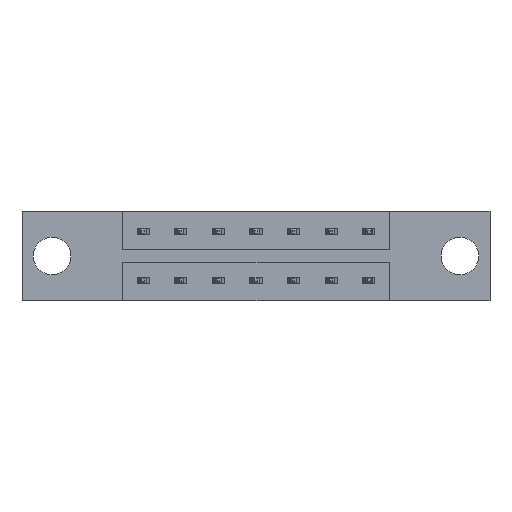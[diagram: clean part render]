
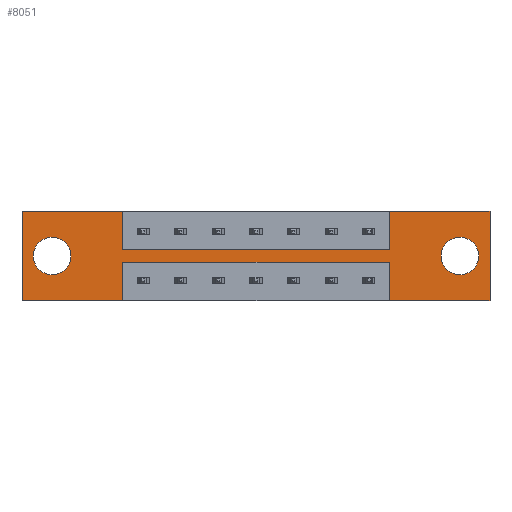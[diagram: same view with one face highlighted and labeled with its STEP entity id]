
A CAD part, front view. The second image highlights one B-rep face of the part: STEP entity #8051.
In plain terms, the highlighted planar face has unit normal (0, -1, 0).
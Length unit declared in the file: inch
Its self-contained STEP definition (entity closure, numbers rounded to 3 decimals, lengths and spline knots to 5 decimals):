
#23 = DIRECTION ( 'NONE',  ( 0., 0., 1. ) ) ;
#122 = DIRECTION ( 'NONE',  ( -1., 0., 0. ) ) ;
#173 = ORIENTED_EDGE ( 'NONE', *, *, #7002, .T. ) ;
#308 = VERTEX_POINT ( 'NONE', #1861 ) ;
#310 = ORIENTED_EDGE ( 'NONE', *, *, #7567, .F. ) ;
#315 = DIRECTION ( 'NONE',  ( 0., 1., 0. ) ) ;
#384 = EDGE_CURVE ( 'NONE', #308, #1176, #7530, .T. ) ;
#392 = ORIENTED_EDGE ( 'NONE', *, *, #9066, .T. ) ;
#439 = VERTEX_POINT ( 'NONE', #3459 ) ;
#445 = EDGE_CURVE ( 'NONE', #5451, #8103, #5532, .T. ) ;
#446 = ORIENTED_EDGE ( 'NONE', *, *, #5977, .F. ) ;
#511 = CIRCLE ( 'NONE', #1690, 0.078 ) ;
#558 = VECTOR ( 'NONE', #1764, 39.37008 ) ;
#586 = LINE ( 'NONE', #7696, #5317 ) ;
#608 = CARTESIAN_POINT ( 'NONE',  ( 0.4175, 0., -0.1585 ) ) ;
#742 = CARTESIAN_POINT ( 'NONE',  ( 0., 0., -0.37 ) ) ;
#937 = CIRCLE ( 'NONE', #1239, 0.078 ) ;
#938 = EDGE_CURVE ( 'NONE', #2151, #2576, #6186, .T. ) ;
#1021 = DIRECTION ( 'NONE',  ( 0., 0., -1. ) ) ;
#1129 = VECTOR ( 'NONE', #5415, 39.37008 ) ;
#1176 = VERTEX_POINT ( 'NONE', #1237 ) ;
#1177 = ORIENTED_EDGE ( 'NONE', *, *, #445, .T. ) ;
#1206 = CARTESIAN_POINT ( 'NONE',  ( 0., 0., -0.37 ) ) ;
#1237 = CARTESIAN_POINT ( 'NONE',  ( 0.4175, 0., -0.1585 ) ) ;
#1239 = AXIS2_PLACEMENT_3D ( 'NONE', #5053, #7260, #5105 ) ;
#1272 = EDGE_CURVE ( 'NONE', #8853, #7526, #586, .T. ) ;
#1282 = ORIENTED_EDGE ( 'NONE', *, *, #1272, .F. ) ;
#1418 = CARTESIAN_POINT ( 'NONE',  ( 1.815, 0., -0.263 ) ) ;
#1430 = EDGE_LOOP ( 'NONE', ( #7044, #6450, #446, #1282, #3227, #310, #8254, #4427, #1470, #2848, #5745, #5926 ) ) ;
#1470 = ORIENTED_EDGE ( 'NONE', *, *, #1856, .F. ) ;
#1485 = CARTESIAN_POINT ( 'NONE',  ( 0.4175, 0., -0.2115 ) ) ;
#1657 = LINE ( 'NONE', #1485, #8416 ) ;
#1690 = AXIS2_PLACEMENT_3D ( 'NONE', #4483, #315, #1021 ) ;
#1727 = VECTOR ( 'NONE', #122, 39.37008 ) ;
#1764 = DIRECTION ( 'NONE',  ( 0., 0., 1. ) ) ;
#1856 = EDGE_CURVE ( 'NONE', #7547, #3653, #6992, .T. ) ;
#1861 = CARTESIAN_POINT ( 'NONE',  ( 0.4175, 0., 0. ) ) ;
#2132 = LINE ( 'NONE', #5685, #6355 ) ;
#2151 = VERTEX_POINT ( 'NONE', #3262 ) ;
#2155 = CARTESIAN_POINT ( 'NONE',  ( 0., 0., -0.37 ) ) ;
#2385 = LINE ( 'NONE', #5078, #8700 ) ;
#2402 = CARTESIAN_POINT ( 'NONE',  ( 0.4175, 0., -0.2115 ) ) ;
#2416 = CARTESIAN_POINT ( 'NONE',  ( 1.815, 0., -0.107 ) ) ;
#2446 = LINE ( 'NONE', #2402, #8591 ) ;
#2576 = VERTEX_POINT ( 'NONE', #5306 ) ;
#2579 = LINE ( 'NONE', #8041, #558 ) ;
#2848 = ORIENTED_EDGE ( 'NONE', *, *, #4275, .F. ) ;
#2861 = CARTESIAN_POINT ( 'NONE',  ( 1.5225, 0., 0. ) ) ;
#2882 = PLANE ( 'NONE',  #6802 ) ;
#2903 = EDGE_CURVE ( 'NONE', #3653, #308, #2385, .T. ) ;
#2936 = LINE ( 'NONE', #6287, #6354 ) ;
#3021 = DIRECTION ( 'NONE',  ( 1., 0., 0. ) ) ;
#3227 = ORIENTED_EDGE ( 'NONE', *, *, #6073, .F. ) ;
#3262 = CARTESIAN_POINT ( 'NONE',  ( 1.94, 0., -0.37 ) ) ;
#3265 = DIRECTION ( 'NONE',  ( 0., 0., 1. ) ) ;
#3439 = FACE_BOUND ( 'NONE', #6124, .T. ) ;
#3459 = CARTESIAN_POINT ( 'NONE',  ( 0.4175, 0., -0.37 ) ) ;
#3562 = DIRECTION ( 'NONE',  ( 0., -1., 0. ) ) ;
#3605 = EDGE_CURVE ( 'NONE', #8575, #439, #2446, .T. ) ;
#3653 = VERTEX_POINT ( 'NONE', #8040 ) ;
#3692 = ORIENTED_EDGE ( 'NONE', *, *, #4993, .T. ) ;
#3773 = VERTEX_POINT ( 'NONE', #8953 ) ;
#3888 = VECTOR ( 'NONE', #6834, 39.37008 ) ;
#4213 = AXIS2_PLACEMENT_3D ( 'NONE', #6888, #7521, #5558 ) ;
#4275 = EDGE_CURVE ( 'NONE', #439, #7547, #4882, .T. ) ;
#4332 = VERTEX_POINT ( 'NONE', #2416 ) ;
#4393 = DIRECTION ( 'NONE',  ( -1., 0., 0. ) ) ;
#4427 = ORIENTED_EDGE ( 'NONE', *, *, #2903, .F. ) ;
#4483 = CARTESIAN_POINT ( 'NONE',  ( 1.815, 0., -0.185 ) ) ;
#4781 = CARTESIAN_POINT ( 'NONE',  ( 1.5225, 0., -0.1585 ) ) ;
#4882 = LINE ( 'NONE', #2155, #1727 ) ;
#4952 = EDGE_CURVE ( 'NONE', #2576, #3773, #2579, .T. ) ;
#4993 = EDGE_CURVE ( 'NONE', #8103, #5451, #5089, .T. ) ;
#5041 = DIRECTION ( 'NONE',  ( 0., 0., 1. ) ) ;
#5053 = CARTESIAN_POINT ( 'NONE',  ( 1.815, 0., -0.185 ) ) ;
#5078 = CARTESIAN_POINT ( 'NONE',  ( 0., 0., 0. ) ) ;
#5089 = CIRCLE ( 'NONE', #4213, 0.078 ) ;
#5105 = DIRECTION ( 'NONE',  ( 0., 0., -1. ) ) ;
#5306 = CARTESIAN_POINT ( 'NONE',  ( 1.5225, 0., -0.37 ) ) ;
#5317 = VECTOR ( 'NONE', #6274, 39.37008 ) ;
#5363 = DIRECTION ( 'NONE',  ( 0., 0., -1. ) ) ;
#5415 = DIRECTION ( 'NONE',  ( 0., 0., -1. ) ) ;
#5451 = VERTEX_POINT ( 'NONE', #8464 ) ;
#5459 = LINE ( 'NONE', #8277, #6944 ) ;
#5515 = CARTESIAN_POINT ( 'NONE',  ( 0.125, 0., -0.185 ) ) ;
#5532 = CIRCLE ( 'NONE', #5797, 0.078 ) ;
#5544 = DIRECTION ( 'NONE',  ( 0., 0., -1. ) ) ;
#5558 = DIRECTION ( 'NONE',  ( 0., 0., 1. ) ) ;
#5560 = DIRECTION ( 'NONE',  ( 0., 0., -1. ) ) ;
#5623 = FACE_OUTER_BOUND ( 'NONE', #1430, .T. ) ;
#5685 = CARTESIAN_POINT ( 'NONE',  ( 1.5225, 0., -0.1585 ) ) ;
#5745 = ORIENTED_EDGE ( 'NONE', *, *, #3605, .F. ) ;
#5797 = AXIS2_PLACEMENT_3D ( 'NONE', #5515, #6983, #3265 ) ;
#5926 = ORIENTED_EDGE ( 'NONE', *, *, #6118, .F. ) ;
#5940 = CARTESIAN_POINT ( 'NONE',  ( 0.125, 0., -0.107 ) ) ;
#5977 = EDGE_CURVE ( 'NONE', #7526, #2151, #5459, .T. ) ;
#6073 = EDGE_CURVE ( 'NONE', #8814, #8853, #2132, .T. ) ;
#6118 = EDGE_CURVE ( 'NONE', #3773, #8575, #1657, .T. ) ;
#6124 = EDGE_LOOP ( 'NONE', ( #173, #392 ) ) ;
#6186 = LINE ( 'NONE', #1206, #3888 ) ;
#6274 = DIRECTION ( 'NONE',  ( 1., 0., 0. ) ) ;
#6287 = CARTESIAN_POINT ( 'NONE',  ( 0.4175, 0., -0.1585 ) ) ;
#6316 = FACE_BOUND ( 'NONE', #7010, .T. ) ;
#6337 = CARTESIAN_POINT ( 'NONE',  ( 0., 0., 0. ) ) ;
#6354 = VECTOR ( 'NONE', #7790, 39.37008 ) ;
#6355 = VECTOR ( 'NONE', #5041, 39.37008 ) ;
#6450 = ORIENTED_EDGE ( 'NONE', *, *, #938, .F. ) ;
#6473 = CARTESIAN_POINT ( 'NONE',  ( 0.4175, 0., -0.2115 ) ) ;
#6780 = CARTESIAN_POINT ( 'NONE',  ( 1.94, 0., 0. ) ) ;
#6802 = AXIS2_PLACEMENT_3D ( 'NONE', #6964, #3562, #5544 ) ;
#6834 = DIRECTION ( 'NONE',  ( -1., 0., 0. ) ) ;
#6888 = CARTESIAN_POINT ( 'NONE',  ( 0.125, 0., -0.185 ) ) ;
#6944 = VECTOR ( 'NONE', #5560, 39.37008 ) ;
#6964 = CARTESIAN_POINT ( 'NONE',  ( 0., 0., -0.37 ) ) ;
#6983 = DIRECTION ( 'NONE',  ( 0., 1., 0. ) ) ;
#6992 = LINE ( 'NONE', #6337, #8497 ) ;
#7002 = EDGE_CURVE ( 'NONE', #4332, #8388, #937, .T. ) ;
#7010 = EDGE_LOOP ( 'NONE', ( #3692, #1177 ) ) ;
#7044 = ORIENTED_EDGE ( 'NONE', *, *, #4952, .F. ) ;
#7260 = DIRECTION ( 'NONE',  ( 0., 1., 0. ) ) ;
#7521 = DIRECTION ( 'NONE',  ( 0., 1., 0. ) ) ;
#7526 = VERTEX_POINT ( 'NONE', #6780 ) ;
#7530 = LINE ( 'NONE', #608, #1129 ) ;
#7547 = VERTEX_POINT ( 'NONE', #742 ) ;
#7567 = EDGE_CURVE ( 'NONE', #1176, #8814, #2936, .T. ) ;
#7696 = CARTESIAN_POINT ( 'NONE',  ( 0., 0., 0. ) ) ;
#7790 = DIRECTION ( 'NONE',  ( 1., 0., 0. ) ) ;
#8040 = CARTESIAN_POINT ( 'NONE',  ( 0., 0., 0. ) ) ;
#8041 = CARTESIAN_POINT ( 'NONE',  ( 1.5225, 0., -0.2115 ) ) ;
#8051 = ADVANCED_FACE ( 'NONE', ( #3439, #6316, #5623 ), #2882, .T. ) ;
#8103 = VERTEX_POINT ( 'NONE', #5940 ) ;
#8254 = ORIENTED_EDGE ( 'NONE', *, *, #384, .F. ) ;
#8277 = CARTESIAN_POINT ( 'NONE',  ( 1.94, 0., 0. ) ) ;
#8388 = VERTEX_POINT ( 'NONE', #1418 ) ;
#8416 = VECTOR ( 'NONE', #4393, 39.37008 ) ;
#8464 = CARTESIAN_POINT ( 'NONE',  ( 0.125, 0., -0.263 ) ) ;
#8497 = VECTOR ( 'NONE', #23, 39.37008 ) ;
#8575 = VERTEX_POINT ( 'NONE', #6473 ) ;
#8591 = VECTOR ( 'NONE', #5363, 39.37008 ) ;
#8700 = VECTOR ( 'NONE', #3021, 39.37008 ) ;
#8814 = VERTEX_POINT ( 'NONE', #4781 ) ;
#8853 = VERTEX_POINT ( 'NONE', #2861 ) ;
#8953 = CARTESIAN_POINT ( 'NONE',  ( 1.5225, 0., -0.2115 ) ) ;
#9066 = EDGE_CURVE ( 'NONE', #8388, #4332, #511, .T. ) ;
